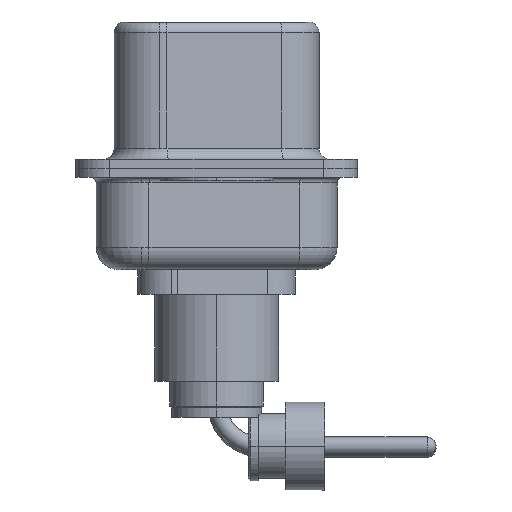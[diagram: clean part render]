
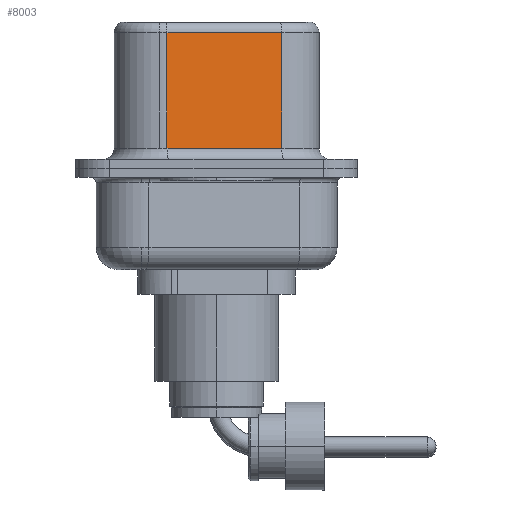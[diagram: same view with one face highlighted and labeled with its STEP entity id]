
A CAD part, left-side view. The second image highlights one B-rep face of the part: STEP entity #8003.
In plain terms, the highlighted planar face has unit normal (-0.985, -0.174, 0).
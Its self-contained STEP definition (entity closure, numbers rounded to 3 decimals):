
#495 = DIRECTION ( 'NONE',  ( 0.985, 0.174, 0. ) ) ;
#962 = EDGE_CURVE ( 'NONE', #9473, #3326, #14317, .T. ) ;
#1862 = FACE_OUTER_BOUND ( 'NONE', #10258, .T. ) ;
#3326 = VERTEX_POINT ( 'NONE', #11939 ) ;
#3340 = ORIENTED_EDGE ( 'NONE', *, *, #16786, .F. ) ;
#3712 = VECTOR ( 'NONE', #4338, 1000. ) ;
#3715 = ORIENTED_EDGE ( 'NONE', *, *, #962, .T. ) ;
#4103 = CARTESIAN_POINT ( 'NONE',  ( 3.655, 2.203, 0.9 ) ) ;
#4338 = DIRECTION ( 'NONE',  ( 0.174, -0.985, 0. ) ) ;
#4634 = DIRECTION ( 'NONE',  ( -0.174, 0.985, 0. ) ) ;
#5341 = LINE ( 'NONE', #5518, #17695 ) ;
#5518 = CARTESIAN_POINT ( 'NONE',  ( 4.555, -2.897, 6.52 ) ) ;
#5955 = LINE ( 'NONE', #8444, #11241 ) ;
#6072 = DIRECTION ( 'NONE',  ( -0.174, 0.985, 0. ) ) ;
#6506 = CARTESIAN_POINT ( 'NONE',  ( 4.555, -2.897, 0.9 ) ) ;
#7320 = ORIENTED_EDGE ( 'NONE', *, *, #8446, .T. ) ;
#7450 = PLANE ( 'NONE',  #8057 ) ;
#8003 = ADVANCED_FACE ( 'NONE', ( #1862 ), #7450, .F. ) ;
#8057 = AXIS2_PLACEMENT_3D ( 'NONE', #13024, #495, #6072 ) ;
#8173 = VERTEX_POINT ( 'NONE', #6506 ) ;
#8444 = CARTESIAN_POINT ( 'NONE',  ( 3.655, 2.203, 6.52 ) ) ;
#8446 = EDGE_CURVE ( 'NONE', #14487, #8173, #14288, .T. ) ;
#9394 = CARTESIAN_POINT ( 'NONE',  ( 4.555, -2.897, 6.02 ) ) ;
#9473 = VERTEX_POINT ( 'NONE', #9394 ) ;
#10258 = EDGE_LOOP ( 'NONE', ( #3340, #3715, #16281, #7320 ) ) ;
#11241 = VECTOR ( 'NONE', #11276, 1000. ) ;
#11276 = DIRECTION ( 'NONE',  ( 0., 0., -1. ) ) ;
#11289 = DIRECTION ( 'NONE',  ( 0., 0., -1. ) ) ;
#11574 = CARTESIAN_POINT ( 'NONE',  ( 4.555, -2.897, 6.02 ) ) ;
#11939 = CARTESIAN_POINT ( 'NONE',  ( 3.655, 2.203, 6.02 ) ) ;
#12998 = CARTESIAN_POINT ( 'NONE',  ( 4.555, -2.897, 0.9 ) ) ;
#13024 = CARTESIAN_POINT ( 'NONE',  ( 4.555, -2.897, 6.52 ) ) ;
#14089 = EDGE_CURVE ( 'NONE', #3326, #14487, #5955, .T. ) ;
#14288 = LINE ( 'NONE', #12998, #3712 ) ;
#14317 = LINE ( 'NONE', #11574, #16571 ) ;
#14487 = VERTEX_POINT ( 'NONE', #4103 ) ;
#16281 = ORIENTED_EDGE ( 'NONE', *, *, #14089, .T. ) ;
#16571 = VECTOR ( 'NONE', #4634, 1000. ) ;
#16786 = EDGE_CURVE ( 'NONE', #9473, #8173, #5341, .T. ) ;
#17695 = VECTOR ( 'NONE', #11289, 1000. ) ;
